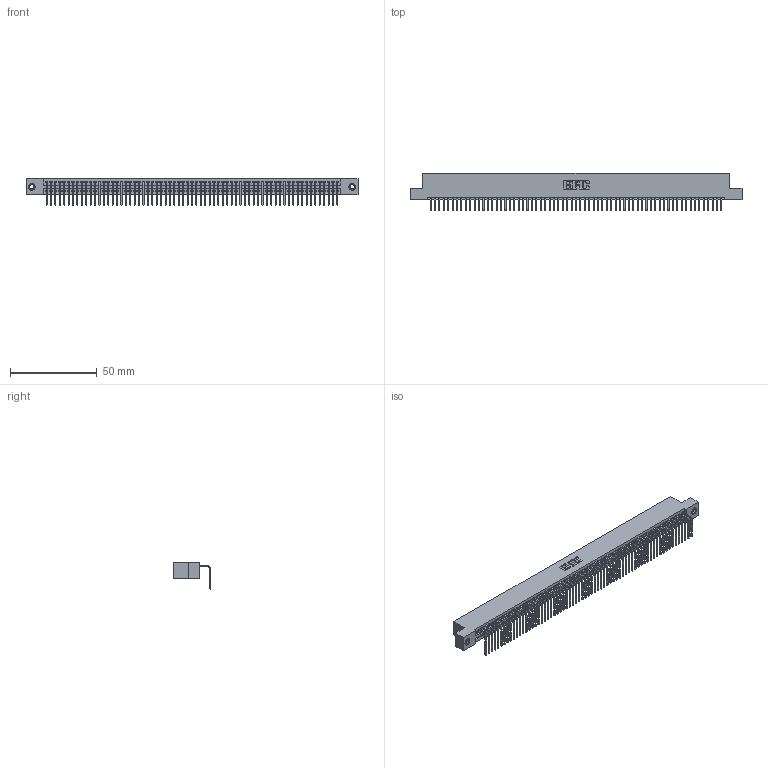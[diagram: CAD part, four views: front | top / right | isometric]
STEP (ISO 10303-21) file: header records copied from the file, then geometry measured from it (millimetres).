
FILE_DESCRIPTION (( 'STEP AP203' ), '1' );
FILE_NAME ('395-067-558-107.STEP', '2018-11-25T11:02:52', ( '' ), ( '' ), 'SwSTEP 2.0', 'SolidWorks 2016', '' );
FILE_SCHEMA (( 'CONFIG_CONTROL_DESIGN' ));
Length unit declared in the file: inch
Products named in the file (4): 395-067-558-107; 345 Part_Flush Mounting Lugs - 0.156 Dia-TI; 345-250-001_345-250-005-103; 345-292-001_558 Tail - 2
Assembly tree (70 placements, depth 2):
  395-067-558-107
    345 Part_Flush Mounting Lugs - 0.156 Dia-TI
    345-292-001_558 Tail - 2  x67
    345-250-001_345-250-005-103  x2
Bounding box: 191.39 x 21.83 x 15.37 mm (x, y, z)
Volume: 18592.8 mm3; surface area: 26392.2 mm2
Topology: 70 solids, 70 shells, 4206 faces, 12671 edges, 8350 vertices
Faces by surface type: plane 2926, cylinder 1264, cone 12, torus 4
Entity records: 48330 total; most frequent: CARTESIAN_POINT 8352, ORIENTED_EDGE 8346, DIRECTION 7285, EDGE_CURVE 4173, LINE 3753, VECTOR 3753, VERTEX_POINT 2776, AXIS2_PLACEMENT_3D 1766
